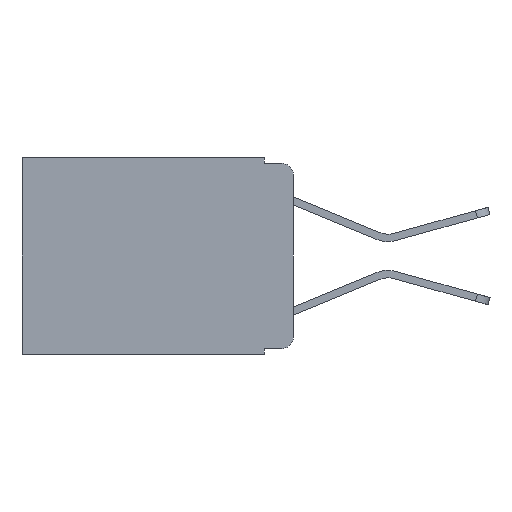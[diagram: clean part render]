
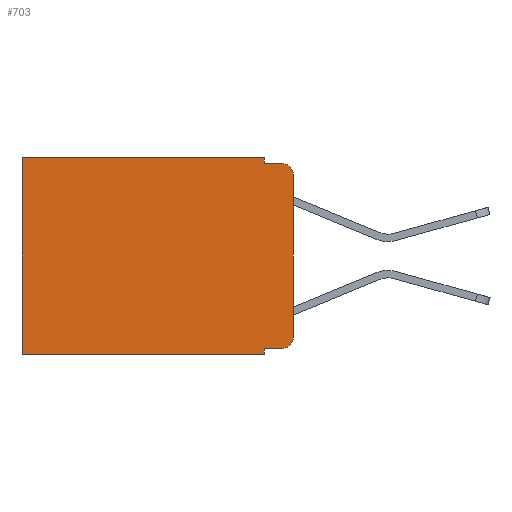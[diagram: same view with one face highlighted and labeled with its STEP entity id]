
A CAD part, left-side view. The second image highlights one B-rep face of the part: STEP entity #703.
In plain terms, the highlighted planar face has unit normal (-1, 0, 0).
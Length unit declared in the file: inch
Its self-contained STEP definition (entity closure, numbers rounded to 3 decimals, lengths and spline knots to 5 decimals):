
#84 = DIRECTION ( 'NONE',  ( 0., -1., 0. ) ) ;
#372 = VERTEX_POINT ( 'NONE', #6377 ) ;
#460 = CARTESIAN_POINT ( 'NONE',  ( 0.298, 0.051, 0. ) ) ;
#496 = VERTEX_POINT ( 'NONE', #8731 ) ;
#583 = LINE ( 'NONE', #5399, #13546 ) ;
#703 = ADVANCED_FACE ( 'NONE', ( #18882 ), #6305, .F. ) ;
#1505 = CARTESIAN_POINT ( 'NONE',  ( 0.298, 0.473, -0.343 ) ) ;
#1772 = DIRECTION ( 'NONE',  ( -1., 0., 0. ) ) ;
#2917 = EDGE_CURVE ( 'NONE', #5979, #20700, #16508, .T. ) ;
#3012 = DIRECTION ( 'NONE',  ( 0., -1., 0. ) ) ;
#3047 = DIRECTION ( 'NONE',  ( 0., 1., 0. ) ) ;
#3073 = CARTESIAN_POINT ( 'NONE',  ( 0.298, 0.051, -0.343 ) ) ;
#3256 = ORIENTED_EDGE ( 'NONE', *, *, #7513, .T. ) ;
#3563 = CARTESIAN_POINT ( 'NONE',  ( 0.298, 0.473, 0. ) ) ;
#3678 = DIRECTION ( 'NONE',  ( 0., 0., -1. ) ) ;
#3726 = VECTOR ( 'NONE', #10798, 39.37008 ) ;
#3838 = EDGE_CURVE ( 'NONE', #8869, #372, #12773, .T. ) ;
#4419 = LINE ( 'NONE', #11975, #13588 ) ;
#4493 = AXIS2_PLACEMENT_3D ( 'NONE', #19737, #21135, #11121 ) ;
#4648 = CARTESIAN_POINT ( 'NONE',  ( 0.298, 0.051, -0.333 ) ) ;
#4971 = CARTESIAN_POINT ( 'NONE',  ( 0.298, 0.051, -0.01 ) ) ;
#5056 = LINE ( 'NONE', #20786, #3726 ) ;
#5195 = CARTESIAN_POINT ( 'NONE',  ( 0.298, 0.02, -0.313 ) ) ;
#5399 = CARTESIAN_POINT ( 'NONE',  ( 0.298, 0., 0. ) ) ;
#5749 = EDGE_CURVE ( 'NONE', #7561, #9111, #5056, .T. ) ;
#5979 = VERTEX_POINT ( 'NONE', #4648 ) ;
#6204 = ORIENTED_EDGE ( 'NONE', *, *, #18179, .F. ) ;
#6305 = PLANE ( 'NONE',  #17430 ) ;
#6377 = CARTESIAN_POINT ( 'NONE',  ( 0.298, 0.02, -0.01 ) ) ;
#6465 = EDGE_CURVE ( 'NONE', #496, #372, #19282, .T. ) ;
#6854 = LINE ( 'NONE', #21617, #11095 ) ;
#7130 = VERTEX_POINT ( 'NONE', #20819 ) ;
#7436 = EDGE_CURVE ( 'NONE', #20700, #9111, #9105, .T. ) ;
#7484 = EDGE_CURVE ( 'NONE', #20698, #7561, #6854, .T. ) ;
#7513 = EDGE_CURVE ( 'NONE', #5979, #7130, #4419, .T. ) ;
#7534 = VECTOR ( 'NONE', #17472, 39.37008 ) ;
#7561 = VERTEX_POINT ( 'NONE', #3563 ) ;
#7575 = EDGE_CURVE ( 'NONE', #7130, #14738, #16181, .T. ) ;
#8731 = CARTESIAN_POINT ( 'NONE',  ( 0.298, 0., -0.03 ) ) ;
#8869 = VERTEX_POINT ( 'NONE', #4971 ) ;
#9036 = CARTESIAN_POINT ( 'NONE',  ( 0.298, 0.051, 0. ) ) ;
#9105 = LINE ( 'NONE', #14836, #21496 ) ;
#9111 = VERTEX_POINT ( 'NONE', #1505 ) ;
#9332 = EDGE_CURVE ( 'NONE', #496, #14738, #583, .T. ) ;
#9500 = CARTESIAN_POINT ( 'NONE',  ( 0.298, 0.051, 0. ) ) ;
#10433 = DIRECTION ( 'NONE',  ( 0., 0., -1. ) ) ;
#10798 = DIRECTION ( 'NONE',  ( 0., 0., -1. ) ) ;
#11095 = VECTOR ( 'NONE', #3047, 39.37008 ) ;
#11121 = DIRECTION ( 'NONE',  ( 0., 0., -1. ) ) ;
#11410 = CARTESIAN_POINT ( 'NONE',  ( 0.298, 0., 0. ) ) ;
#11595 = ORIENTED_EDGE ( 'NONE', *, *, #2917, .F. ) ;
#11716 = CARTESIAN_POINT ( 'NONE',  ( 0.298, 0., -0.313 ) ) ;
#11975 = CARTESIAN_POINT ( 'NONE',  ( 0.298, 0.051, -0.333 ) ) ;
#12773 = LINE ( 'NONE', #13121, #18865 ) ;
#12968 = AXIS2_PLACEMENT_3D ( 'NONE', #5195, #1772, #10433 ) ;
#13045 = ORIENTED_EDGE ( 'NONE', *, *, #7484, .T. ) ;
#13121 = CARTESIAN_POINT ( 'NONE',  ( 0.298, 0.051, -0.01 ) ) ;
#13426 = ORIENTED_EDGE ( 'NONE', *, *, #7436, .F. ) ;
#13546 = VECTOR ( 'NONE', #3678, 39.37008 ) ;
#13588 = VECTOR ( 'NONE', #84, 39.37008 ) ;
#13913 = DIRECTION ( 'NONE',  ( 0., 0., -1. ) ) ;
#14249 = EDGE_LOOP ( 'NONE', ( #16120, #14297, #14553, #6204, #13045, #16594, #13426, #11595, #3256, #18049 ) ) ;
#14297 = ORIENTED_EDGE ( 'NONE', *, *, #6465, .T. ) ;
#14352 = LINE ( 'NONE', #9036, #17295 ) ;
#14553 = ORIENTED_EDGE ( 'NONE', *, *, #3838, .F. ) ;
#14738 = VERTEX_POINT ( 'NONE', #11716 ) ;
#14836 = CARTESIAN_POINT ( 'NONE',  ( 0.298, 0., -0.343 ) ) ;
#16120 = ORIENTED_EDGE ( 'NONE', *, *, #9332, .F. ) ;
#16181 = CIRCLE ( 'NONE', #12968, 0.02 ) ;
#16508 = LINE ( 'NONE', #460, #7534 ) ;
#16594 = ORIENTED_EDGE ( 'NONE', *, *, #5749, .T. ) ;
#17295 = VECTOR ( 'NONE', #13913, 39.37008 ) ;
#17430 = AXIS2_PLACEMENT_3D ( 'NONE', #11410, #18146, #19798 ) ;
#17472 = DIRECTION ( 'NONE',  ( 0., 0., -1. ) ) ;
#18049 = ORIENTED_EDGE ( 'NONE', *, *, #7575, .T. ) ;
#18146 = DIRECTION ( 'NONE',  ( 1., 0., 0. ) ) ;
#18179 = EDGE_CURVE ( 'NONE', #20698, #8869, #14352, .T. ) ;
#18865 = VECTOR ( 'NONE', #3012, 39.37008 ) ;
#18882 = FACE_OUTER_BOUND ( 'NONE', #14249, .T. ) ;
#19282 = CIRCLE ( 'NONE', #4493, 0.02 ) ;
#19737 = CARTESIAN_POINT ( 'NONE',  ( 0.298, 0.02, -0.03 ) ) ;
#19798 = DIRECTION ( 'NONE',  ( 0., 0., -1. ) ) ;
#20698 = VERTEX_POINT ( 'NONE', #9500 ) ;
#20700 = VERTEX_POINT ( 'NONE', #3073 ) ;
#20786 = CARTESIAN_POINT ( 'NONE',  ( 0.298, 0.473, 0. ) ) ;
#20819 = CARTESIAN_POINT ( 'NONE',  ( 0.298, 0.02, -0.333 ) ) ;
#21135 = DIRECTION ( 'NONE',  ( -1., 0., 0. ) ) ;
#21496 = VECTOR ( 'NONE', #21697, 39.37008 ) ;
#21617 = CARTESIAN_POINT ( 'NONE',  ( 0.298, 0., 0. ) ) ;
#21697 = DIRECTION ( 'NONE',  ( 0., 1., 0. ) ) ;
